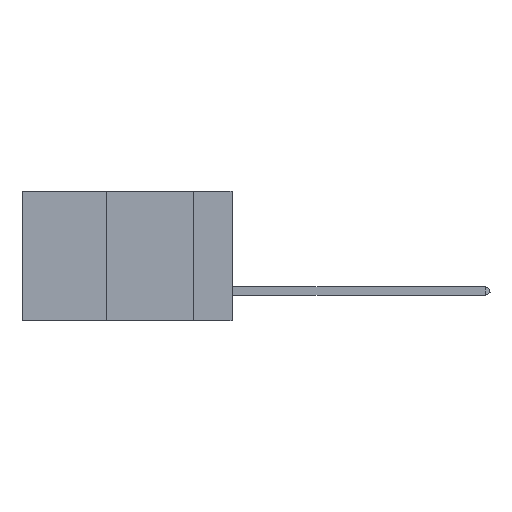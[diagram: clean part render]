
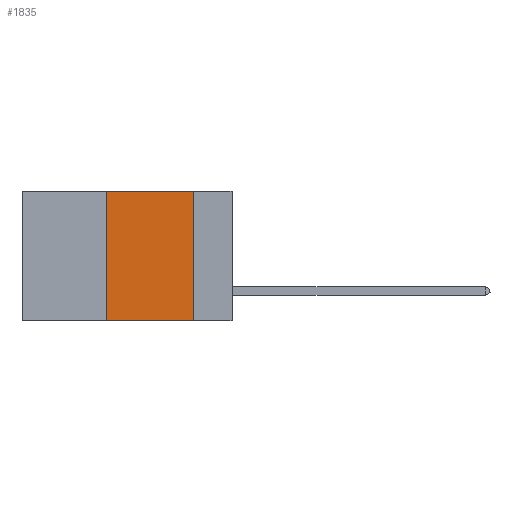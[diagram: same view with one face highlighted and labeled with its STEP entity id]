
A CAD part, left-side view. The second image highlights one B-rep face of the part: STEP entity #1835.
In plain terms, the highlighted planar face has unit normal (-1, 0, 0).
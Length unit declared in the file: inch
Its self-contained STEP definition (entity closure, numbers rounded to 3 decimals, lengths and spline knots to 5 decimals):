
#458 = CARTESIAN_POINT ( 'NONE',  ( 0., 0.36, -0.37 ) ) ;
#1307 = ORIENTED_EDGE ( 'NONE', *, *, #12700, .F. ) ;
#1793 = CARTESIAN_POINT ( 'NONE',  ( 0., 0.11, 0. ) ) ;
#1835 = ADVANCED_FACE ( 'NONE', ( #11518 ), #6545, .F. ) ;
#2410 = CARTESIAN_POINT ( 'NONE',  ( 0., 0.11, 0. ) ) ;
#4480 = DIRECTION ( 'NONE',  ( 0., 0., 1. ) ) ;
#4584 = EDGE_CURVE ( 'NONE', #11692, #19273, #21726, .T. ) ;
#4650 = VECTOR ( 'NONE', #13167, 39.37008 ) ;
#4777 = VECTOR ( 'NONE', #9467, 39.37008 ) ;
#5581 = LINE ( 'NONE', #17876, #21761 ) ;
#6301 = CARTESIAN_POINT ( 'NONE',  ( 0., 0.6, 0. ) ) ;
#6545 = PLANE ( 'NONE',  #18233 ) ;
#7591 = ORIENTED_EDGE ( 'NONE', *, *, #11621, .T. ) ;
#9216 = ORIENTED_EDGE ( 'NONE', *, *, #10897, .F. ) ;
#9467 = DIRECTION ( 'NONE',  ( 0., 0., -1. ) ) ;
#9998 = DIRECTION ( 'NONE',  ( 1., 0., 0. ) ) ;
#10897 = EDGE_CURVE ( 'NONE', #24312, #11692, #14113, .T. ) ;
#11518 = FACE_OUTER_BOUND ( 'NONE', #19914, .T. ) ;
#11621 = EDGE_CURVE ( 'NONE', #24312, #16568, #5581, .T. ) ;
#11666 = ORIENTED_EDGE ( 'NONE', *, *, #4584, .F. ) ;
#11667 = DIRECTION ( 'NONE',  ( 0., -1., 0. ) ) ;
#11692 = VERTEX_POINT ( 'NONE', #19079 ) ;
#12700 = EDGE_CURVE ( 'NONE', #19273, #16568, #15329, .T. ) ;
#13167 = DIRECTION ( 'NONE',  ( 0., -1., 0. ) ) ;
#13808 = VECTOR ( 'NONE', #4480, 39.37008 ) ;
#14113 = LINE ( 'NONE', #23315, #13808 ) ;
#15324 = CARTESIAN_POINT ( 'NONE',  ( 0., 0.6, 0. ) ) ;
#15329 = LINE ( 'NONE', #1793, #4777 ) ;
#15551 = DIRECTION ( 'NONE',  ( 0., 0., -1. ) ) ;
#16568 = VERTEX_POINT ( 'NONE', #21972 ) ;
#17876 = CARTESIAN_POINT ( 'NONE',  ( 0., 0.6, -0.37 ) ) ;
#18233 = AXIS2_PLACEMENT_3D ( 'NONE', #6301, #9998, #15551 ) ;
#19079 = CARTESIAN_POINT ( 'NONE',  ( 0., 0.36, 0. ) ) ;
#19273 = VERTEX_POINT ( 'NONE', #2410 ) ;
#19914 = EDGE_LOOP ( 'NONE', ( #1307, #11666, #9216, #7591 ) ) ;
#21726 = LINE ( 'NONE', #15324, #4650 ) ;
#21761 = VECTOR ( 'NONE', #11667, 39.37008 ) ;
#21972 = CARTESIAN_POINT ( 'NONE',  ( 0., 0.11, -0.37 ) ) ;
#23315 = CARTESIAN_POINT ( 'NONE',  ( 0., 0.36, 0. ) ) ;
#24312 = VERTEX_POINT ( 'NONE', #458 ) ;
